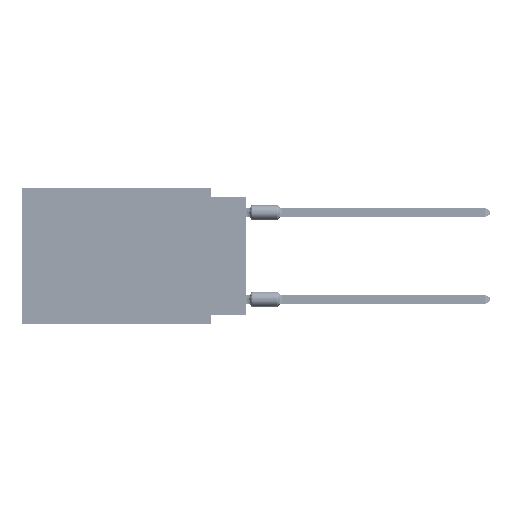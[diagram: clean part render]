
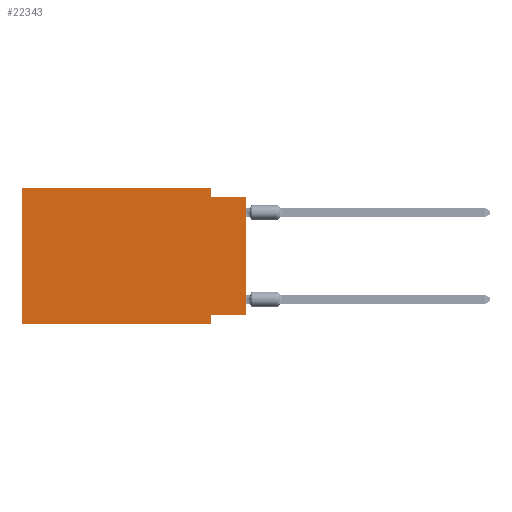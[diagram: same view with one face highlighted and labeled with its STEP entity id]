
A CAD part, left-side view. The second image highlights one B-rep face of the part: STEP entity #22343.
In plain terms, the highlighted planar face has unit normal (-1, 0, 0).
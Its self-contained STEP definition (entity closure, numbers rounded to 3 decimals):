
#308 = VECTOR ( 'NONE', #74084, 1000. ) ;
#1588 = PLANE ( 'NONE',  #71943 ) ;
#3114 = ORIENTED_EDGE ( 'NONE', *, *, #33798, .T. ) ;
#3435 = CARTESIAN_POINT ( 'NONE',  ( 0., 16.383, 0. ) ) ;
#5504 = ORIENTED_EDGE ( 'NONE', *, *, #28581, .F. ) ;
#6160 = CARTESIAN_POINT ( 'NONE',  ( 0., 16.383, -9.906 ) ) ;
#6552 = CARTESIAN_POINT ( 'NONE',  ( 0., 0., -0.635 ) ) ;
#7603 = CARTESIAN_POINT ( 'NONE',  ( 0., 2.54, 0. ) ) ;
#11725 = CARTESIAN_POINT ( 'NONE',  ( 0., 2.54, -0.635 ) ) ;
#13547 = CARTESIAN_POINT ( 'NONE',  ( 0., 0., 0. ) ) ;
#14207 = ORIENTED_EDGE ( 'NONE', *, *, #82094, .T. ) ;
#17690 = ORIENTED_EDGE ( 'NONE', *, *, #33730, .F. ) ;
#19891 = LINE ( 'NONE', #20312, #49545 ) ;
#20066 = DIRECTION ( 'NONE',  ( 0., 0., 1. ) ) ;
#20246 = CARTESIAN_POINT ( 'NONE',  ( 0., 16.383, -9.906 ) ) ;
#20312 = CARTESIAN_POINT ( 'NONE',  ( 0., 0., -9.271 ) ) ;
#20330 = EDGE_CURVE ( 'NONE', #67721, #43631, #19891, .T. ) ;
#22343 = ADVANCED_FACE ( 'NONE', ( #35873 ), #1588, .F. ) ;
#23571 = ORIENTED_EDGE ( 'NONE', *, *, #67425, .F. ) ;
#25071 = CARTESIAN_POINT ( 'NONE',  ( 0., 0., -0.635 ) ) ;
#27603 = VERTEX_POINT ( 'NONE', #6160 ) ;
#28069 = DIRECTION ( 'NONE',  ( 0., 0., -1. ) ) ;
#28581 = EDGE_CURVE ( 'NONE', #43631, #60599, #64314, .T. ) ;
#31582 = DIRECTION ( 'NONE',  ( 0., -1., 0. ) ) ;
#32104 = VECTOR ( 'NONE', #75563, 1000. ) ;
#32829 = CARTESIAN_POINT ( 'NONE',  ( 0., 16.383, 0. ) ) ;
#33135 = EDGE_CURVE ( 'NONE', #50384, #67792, #62097, .T. ) ;
#33730 = EDGE_CURVE ( 'NONE', #27603, #50384, #38059, .T. ) ;
#33798 = EDGE_CURVE ( 'NONE', #27603, #60599, #79306, .T. ) ;
#35873 = FACE_OUTER_BOUND ( 'NONE', #69244, .T. ) ;
#38059 = LINE ( 'NONE', #32829, #77936 ) ;
#38954 = ORIENTED_EDGE ( 'NONE', *, *, #33135, .F. ) ;
#39136 = DIRECTION ( 'NONE',  ( 0., 0., -1. ) ) ;
#41778 = CARTESIAN_POINT ( 'NONE',  ( 0., 0., -9.271 ) ) ;
#43631 = VERTEX_POINT ( 'NONE', #52361 ) ;
#44820 = CARTESIAN_POINT ( 'NONE',  ( 0., 2.54, -9.906 ) ) ;
#48246 = LINE ( 'NONE', #13547, #75825 ) ;
#49545 = VECTOR ( 'NONE', #78947, 1000. ) ;
#50384 = VERTEX_POINT ( 'NONE', #3435 ) ;
#52361 = CARTESIAN_POINT ( 'NONE',  ( 0., 2.54, -9.271 ) ) ;
#52378 = DIRECTION ( 'NONE',  ( 0., 0., 1. ) ) ;
#55403 = CARTESIAN_POINT ( 'NONE',  ( 0., 16.383, 0. ) ) ;
#58914 = EDGE_CURVE ( 'NONE', #75815, #71904, #71115, .T. ) ;
#59110 = CARTESIAN_POINT ( 'NONE',  ( 0., 2.54, -9.906 ) ) ;
#59672 = ORIENTED_EDGE ( 'NONE', *, *, #20330, .F. ) ;
#60599 = VERTEX_POINT ( 'NONE', #44820 ) ;
#62097 = LINE ( 'NONE', #82079, #32104 ) ;
#64314 = LINE ( 'NONE', #59110, #77398 ) ;
#67077 = LINE ( 'NONE', #7603, #74934 ) ;
#67425 = EDGE_CURVE ( 'NONE', #67792, #75815, #67077, .T. ) ;
#67721 = VERTEX_POINT ( 'NONE', #41778 ) ;
#67792 = VERTEX_POINT ( 'NONE', #76515 ) ;
#68354 = VECTOR ( 'NONE', #31582, 1000. ) ;
#69244 = EDGE_LOOP ( 'NONE', ( #14207, #74311, #23571, #38954, #17690, #3114, #5504, #59672 ) ) ;
#71115 = LINE ( 'NONE', #25071, #68354 ) ;
#71904 = VERTEX_POINT ( 'NONE', #6552 ) ;
#71943 = AXIS2_PLACEMENT_3D ( 'NONE', #55403, #75405, #28069 ) ;
#74084 = DIRECTION ( 'NONE',  ( 0., -1., 0. ) ) ;
#74311 = ORIENTED_EDGE ( 'NONE', *, *, #58914, .F. ) ;
#74934 = VECTOR ( 'NONE', #80122, 1000. ) ;
#75405 = DIRECTION ( 'NONE',  ( 1., 0., 0. ) ) ;
#75563 = DIRECTION ( 'NONE',  ( 0., -1., 0. ) ) ;
#75815 = VERTEX_POINT ( 'NONE', #11725 ) ;
#75825 = VECTOR ( 'NONE', #20066, 1000. ) ;
#76515 = CARTESIAN_POINT ( 'NONE',  ( 0., 2.54, 0. ) ) ;
#77398 = VECTOR ( 'NONE', #39136, 1000. ) ;
#77936 = VECTOR ( 'NONE', #52378, 1000. ) ;
#78947 = DIRECTION ( 'NONE',  ( 0., 1., 0. ) ) ;
#79306 = LINE ( 'NONE', #20246, #308 ) ;
#80122 = DIRECTION ( 'NONE',  ( 0., 0., -1. ) ) ;
#82079 = CARTESIAN_POINT ( 'NONE',  ( 0., 16.383, 0. ) ) ;
#82094 = EDGE_CURVE ( 'NONE', #67721, #71904, #48246, .T. ) ;
